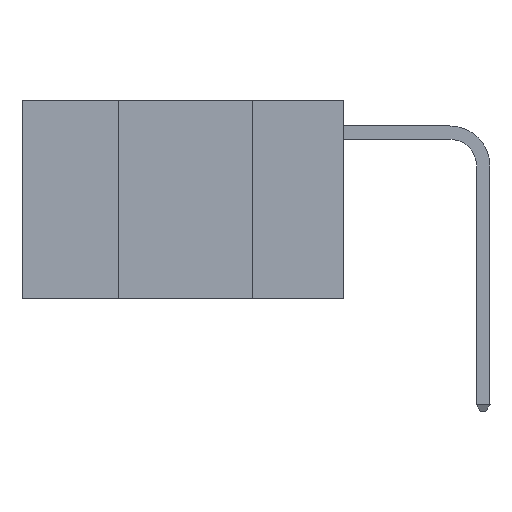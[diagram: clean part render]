
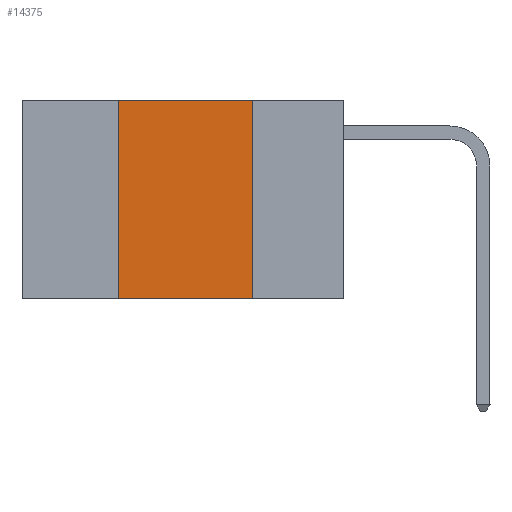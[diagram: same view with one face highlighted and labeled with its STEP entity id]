
A CAD part, left-side view. The second image highlights one B-rep face of the part: STEP entity #14375.
In plain terms, the highlighted planar face has unit normal (-1, 0, 0).
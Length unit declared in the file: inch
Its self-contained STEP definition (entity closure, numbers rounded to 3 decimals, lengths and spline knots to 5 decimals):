
#991 = PLANE ( 'NONE',  #19851 ) ;
#2643 = EDGE_CURVE ( 'NONE', #27873, #22876, #10262, .T. ) ;
#2845 = ORIENTED_EDGE ( 'NONE', *, *, #26503, .T. ) ;
#3915 = ORIENTED_EDGE ( 'NONE', *, *, #27938, .F. ) ;
#3923 = ORIENTED_EDGE ( 'NONE', *, *, #2643, .F. ) ;
#5519 = CARTESIAN_POINT ( 'NONE',  ( 0., 0.17, 0. ) ) ;
#5800 = CARTESIAN_POINT ( 'NONE',  ( 0., 0.6, 0. ) ) ;
#6109 = VECTOR ( 'NONE', #10671, 39.37008 ) ;
#8152 = EDGE_LOOP ( 'NONE', ( #26578, #3915, #3923, #2845 ) ) ;
#8325 = FACE_OUTER_BOUND ( 'NONE', #8152, .T. ) ;
#10262 = LINE ( 'NONE', #12394, #10515 ) ;
#10410 = LINE ( 'NONE', #19705, #17806 ) ;
#10515 = VECTOR ( 'NONE', #21249, 39.37008 ) ;
#10551 = DIRECTION ( 'NONE',  ( 0., -1., 0. ) ) ;
#10671 = DIRECTION ( 'NONE',  ( 0., -1., 0. ) ) ;
#12394 = CARTESIAN_POINT ( 'NONE',  ( 0., 0.42, 0. ) ) ;
#13511 = VECTOR ( 'NONE', #16803, 39.37008 ) ;
#14375 = ADVANCED_FACE ( 'NONE', ( #8325 ), #991, .F. ) ;
#15407 = EDGE_CURVE ( 'NONE', #23370, #20592, #16949, .T. ) ;
#16803 = DIRECTION ( 'NONE',  ( 0., 0., -1. ) ) ;
#16949 = LINE ( 'NONE', #5519, #13511 ) ;
#17616 = CARTESIAN_POINT ( 'NONE',  ( 0., 0.6, 0. ) ) ;
#17806 = VECTOR ( 'NONE', #10551, 39.37008 ) ;
#19027 = CARTESIAN_POINT ( 'NONE',  ( 0., 0.42, 0. ) ) ;
#19390 = CARTESIAN_POINT ( 'NONE',  ( 0., 0.17, 0. ) ) ;
#19705 = CARTESIAN_POINT ( 'NONE',  ( 0., 0.6, -0.37 ) ) ;
#19851 = AXIS2_PLACEMENT_3D ( 'NONE', #17616, #22322, #23575 ) ;
#20592 = VERTEX_POINT ( 'NONE', #28725 ) ;
#21249 = DIRECTION ( 'NONE',  ( 0., 0., 1. ) ) ;
#22322 = DIRECTION ( 'NONE',  ( 1., 0., 0. ) ) ;
#22876 = VERTEX_POINT ( 'NONE', #19027 ) ;
#23370 = VERTEX_POINT ( 'NONE', #19390 ) ;
#23575 = DIRECTION ( 'NONE',  ( 0., 0., -1. ) ) ;
#23767 = CARTESIAN_POINT ( 'NONE',  ( 0., 0.42, -0.37 ) ) ;
#26503 = EDGE_CURVE ( 'NONE', #27873, #20592, #10410, .T. ) ;
#26578 = ORIENTED_EDGE ( 'NONE', *, *, #15407, .F. ) ;
#27245 = LINE ( 'NONE', #5800, #6109 ) ;
#27873 = VERTEX_POINT ( 'NONE', #23767 ) ;
#27938 = EDGE_CURVE ( 'NONE', #22876, #23370, #27245, .T. ) ;
#28725 = CARTESIAN_POINT ( 'NONE',  ( 0., 0.17, -0.37 ) ) ;
